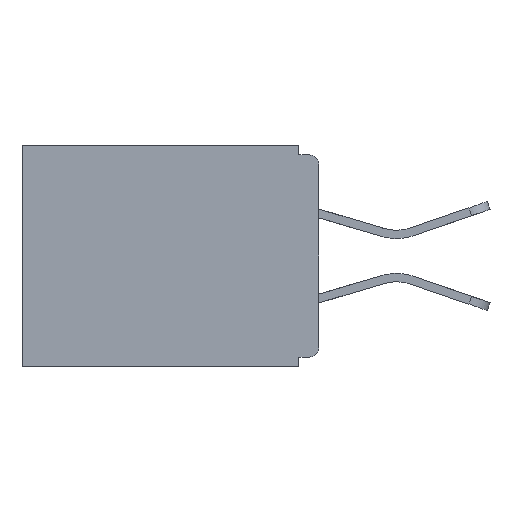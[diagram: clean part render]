
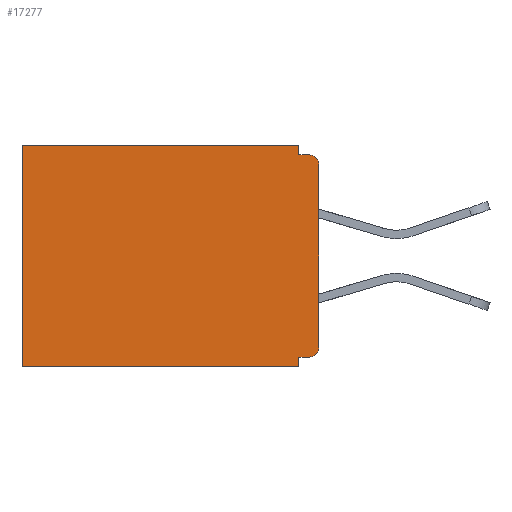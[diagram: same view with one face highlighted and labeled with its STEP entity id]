
A CAD part, left-side view. The second image highlights one B-rep face of the part: STEP entity #17277.
In plain terms, the highlighted planar face has unit normal (-1, 0, 0).
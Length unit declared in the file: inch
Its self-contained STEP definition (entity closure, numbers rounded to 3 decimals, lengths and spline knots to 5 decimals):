
#122 = DIRECTION ( 'NONE',  ( 0., 0., -1. ) ) ;
#144 = DIRECTION ( 'NONE',  ( 0., 1., 0. ) ) ;
#1425 = ORIENTED_EDGE ( 'NONE', *, *, #10547, .T. ) ;
#1677 = EDGE_CURVE ( 'NONE', #8369, #4944, #10496, .T. ) ;
#1930 = ORIENTED_EDGE ( 'NONE', *, *, #5794, .F. ) ;
#2646 = PLANE ( 'NONE',  #15510 ) ;
#3115 = DIRECTION ( 'NONE',  ( 0., 0., -1. ) ) ;
#3381 = EDGE_CURVE ( 'NONE', #19171, #7340, #4590, .T. ) ;
#4033 = DIRECTION ( 'NONE',  ( 0., 1., 0. ) ) ;
#4433 = CARTESIAN_POINT ( 'NONE',  ( 0.298, 0., 0. ) ) ;
#4590 = LINE ( 'NONE', #16001, #18016 ) ;
#4660 = DIRECTION ( 'NONE',  ( 0., 0., -1. ) ) ;
#4944 = VERTEX_POINT ( 'NONE', #13562 ) ;
#5317 = LINE ( 'NONE', #21016, #17371 ) ;
#5376 = ORIENTED_EDGE ( 'NONE', *, *, #16057, .F. ) ;
#5794 = EDGE_CURVE ( 'NONE', #21110, #19062, #5317, .T. ) ;
#5960 = DIRECTION ( 'NONE',  ( 0., 0., -1. ) ) ;
#5993 = VECTOR ( 'NONE', #3115, 39.37008 ) ;
#6058 = DIRECTION ( 'NONE',  ( 0., 1., 0. ) ) ;
#6324 = EDGE_CURVE ( 'NONE', #19171, #21197, #18696, .T. ) ;
#7016 = LINE ( 'NONE', #18912, #15434 ) ;
#7340 = VERTEX_POINT ( 'NONE', #21522 ) ;
#7589 = ORIENTED_EDGE ( 'NONE', *, *, #14499, .T. ) ;
#7818 = ORIENTED_EDGE ( 'NONE', *, *, #3381, .F. ) ;
#8369 = VERTEX_POINT ( 'NONE', #18262 ) ;
#8400 = EDGE_LOOP ( 'NONE', ( #1425, #5376, #7818, #14340, #7589, #1930, #20097, #9678, #15565, #14359 ) ) ;
#8677 = VECTOR ( 'NONE', #6058, 39.37008 ) ;
#8694 = CARTESIAN_POINT ( 'NONE',  ( 0.298, 0.015, -0.328 ) ) ;
#8803 = CIRCLE ( 'NONE', #18333, 0.015 ) ;
#8883 = CARTESIAN_POINT ( 'NONE',  ( 0.298, 0.46, 0. ) ) ;
#9678 = ORIENTED_EDGE ( 'NONE', *, *, #10443, .F. ) ;
#9952 = VECTOR ( 'NONE', #10093, 39.37008 ) ;
#10093 = DIRECTION ( 'NONE',  ( 0., 0., -1. ) ) ;
#10443 = EDGE_CURVE ( 'NONE', #19917, #16937, #7016, .T. ) ;
#10496 = LINE ( 'NONE', #20059, #5993 ) ;
#10547 = EDGE_CURVE ( 'NONE', #8369, #13446, #14088, .T. ) ;
#11082 = VECTOR ( 'NONE', #13007, 39.37008 ) ;
#11341 = EDGE_CURVE ( 'NONE', #19917, #4944, #8803, .T. ) ;
#12571 = LINE ( 'NONE', #17016, #9952 ) ;
#13007 = DIRECTION ( 'NONE',  ( 0., 0., -1. ) ) ;
#13008 = CARTESIAN_POINT ( 'NONE',  ( 0.298, 0.015, -0.03 ) ) ;
#13446 = VERTEX_POINT ( 'NONE', #15512 ) ;
#13562 = CARTESIAN_POINT ( 'NONE',  ( 0.298, 0., -0.313 ) ) ;
#14088 = CIRCLE ( 'NONE', #20024, 0.015 ) ;
#14298 = CARTESIAN_POINT ( 'NONE',  ( 0.298, 0.031, -0.343 ) ) ;
#14340 = ORIENTED_EDGE ( 'NONE', *, *, #6324, .T. ) ;
#14359 = ORIENTED_EDGE ( 'NONE', *, *, #1677, .F. ) ;
#14388 = FACE_OUTER_BOUND ( 'NONE', #8400, .T. ) ;
#14499 = EDGE_CURVE ( 'NONE', #21197, #19062, #15559, .T. ) ;
#15093 = CARTESIAN_POINT ( 'NONE',  ( 0.298, 0.015, -0.313 ) ) ;
#15434 = VECTOR ( 'NONE', #144, 39.37008 ) ;
#15510 = AXIS2_PLACEMENT_3D ( 'NONE', #15864, #21180, #20894 ) ;
#15512 = CARTESIAN_POINT ( 'NONE',  ( 0.298, 0.015, -0.015 ) ) ;
#15559 = LINE ( 'NONE', #8883, #11082 ) ;
#15565 = ORIENTED_EDGE ( 'NONE', *, *, #11341, .T. ) ;
#15864 = CARTESIAN_POINT ( 'NONE',  ( 0.298, 0., 0. ) ) ;
#15992 = VECTOR ( 'NONE', #18581, 39.37008 ) ;
#16001 = CARTESIAN_POINT ( 'NONE',  ( 0.298, 0.031, -0.343 ) ) ;
#16057 = EDGE_CURVE ( 'NONE', #7340, #13446, #20522, .T. ) ;
#16231 = CARTESIAN_POINT ( 'NONE',  ( 0.298, 0.46, -0.343 ) ) ;
#16613 = CARTESIAN_POINT ( 'NONE',  ( 0.298, 0.031, 0. ) ) ;
#16802 = DIRECTION ( 'NONE',  ( -1., 0., 0. ) ) ;
#16937 = VERTEX_POINT ( 'NONE', #19980 ) ;
#17016 = CARTESIAN_POINT ( 'NONE',  ( 0.298, 0.031, -0.343 ) ) ;
#17277 = ADVANCED_FACE ( 'NONE', ( #14388 ), #2646, .F. ) ;
#17371 = VECTOR ( 'NONE', #4033, 39.37008 ) ;
#18016 = VECTOR ( 'NONE', #5960, 39.37008 ) ;
#18123 = DIRECTION ( 'NONE',  ( -1., 0., 0. ) ) ;
#18262 = CARTESIAN_POINT ( 'NONE',  ( 0.298, 0., -0.03 ) ) ;
#18333 = AXIS2_PLACEMENT_3D ( 'NONE', #15093, #16802, #122 ) ;
#18581 = DIRECTION ( 'NONE',  ( 0., -1., 0. ) ) ;
#18696 = LINE ( 'NONE', #4433, #8677 ) ;
#18912 = CARTESIAN_POINT ( 'NONE',  ( 0.298, 0., -0.328 ) ) ;
#19062 = VERTEX_POINT ( 'NONE', #16231 ) ;
#19171 = VERTEX_POINT ( 'NONE', #16613 ) ;
#19917 = VERTEX_POINT ( 'NONE', #8694 ) ;
#19980 = CARTESIAN_POINT ( 'NONE',  ( 0.298, 0.031, -0.328 ) ) ;
#20024 = AXIS2_PLACEMENT_3D ( 'NONE', #13008, #18123, #4660 ) ;
#20059 = CARTESIAN_POINT ( 'NONE',  ( 0.298, 0., 0. ) ) ;
#20097 = ORIENTED_EDGE ( 'NONE', *, *, #20950, .F. ) ;
#20522 = LINE ( 'NONE', #21656, #15992 ) ;
#20894 = DIRECTION ( 'NONE',  ( 0., 0., -1. ) ) ;
#20950 = EDGE_CURVE ( 'NONE', #16937, #21110, #12571, .T. ) ;
#20961 = CARTESIAN_POINT ( 'NONE',  ( 0.298, 0.46, 0. ) ) ;
#21016 = CARTESIAN_POINT ( 'NONE',  ( 0.298, 0., -0.343 ) ) ;
#21110 = VERTEX_POINT ( 'NONE', #14298 ) ;
#21180 = DIRECTION ( 'NONE',  ( 1., 0., 0. ) ) ;
#21197 = VERTEX_POINT ( 'NONE', #20961 ) ;
#21522 = CARTESIAN_POINT ( 'NONE',  ( 0.298, 0.031, -0.015 ) ) ;
#21656 = CARTESIAN_POINT ( 'NONE',  ( 0.298, 0., -0.015 ) ) ;
